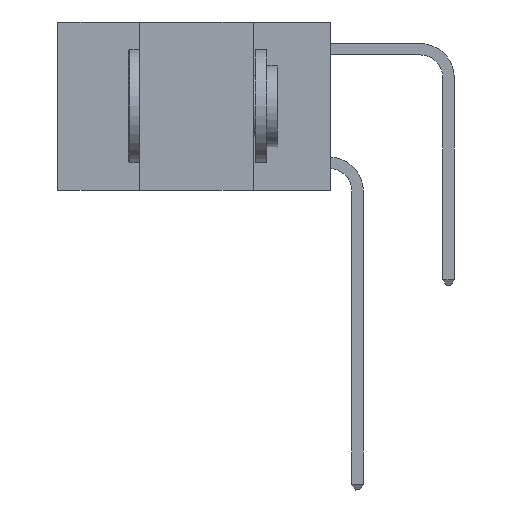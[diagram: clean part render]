
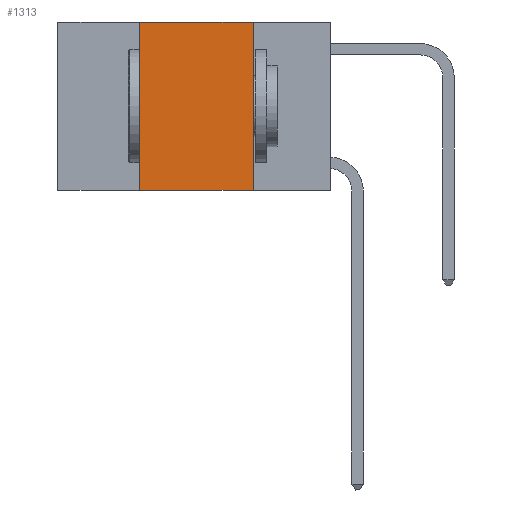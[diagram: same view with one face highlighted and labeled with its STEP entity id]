
A CAD part, left-side view. The second image highlights one B-rep face of the part: STEP entity #1313.
In plain terms, the highlighted planar face has unit normal (-1, 0, 0).
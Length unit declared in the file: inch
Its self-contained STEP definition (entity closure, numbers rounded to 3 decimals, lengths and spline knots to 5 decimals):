
#328 = EDGE_CURVE ( 'NONE', #8473, #8412, #13324, .T. ) ;
#923 = CARTESIAN_POINT ( 'NONE',  ( 0., 0.6, 0. ) ) ;
#1313 = ADVANCED_FACE ( 'NONE', ( #15632 ), #5623, .F. ) ;
#1530 = ORIENTED_EDGE ( 'NONE', *, *, #328, .F. ) ;
#1675 = VECTOR ( 'NONE', #2755, 39.37008 ) ;
#1776 = VECTOR ( 'NONE', #9753, 39.37008 ) ;
#2530 = LINE ( 'NONE', #5169, #1675 ) ;
#2643 = CARTESIAN_POINT ( 'NONE',  ( 0., 0.42, 0. ) ) ;
#2755 = DIRECTION ( 'NONE',  ( 0., 0., 1. ) ) ;
#3214 = DIRECTION ( 'NONE',  ( 0., 0., -1. ) ) ;
#4491 = EDGE_CURVE ( 'NONE', #8412, #13596, #15709, .T. ) ;
#4605 = CARTESIAN_POINT ( 'NONE',  ( 0., 0.17, -0.37 ) ) ;
#5169 = CARTESIAN_POINT ( 'NONE',  ( 0., 0.42, 0. ) ) ;
#5623 = PLANE ( 'NONE',  #15043 ) ;
#6271 = CARTESIAN_POINT ( 'NONE',  ( 0., 0.17, 0. ) ) ;
#6325 = EDGE_CURVE ( 'NONE', #7435, #8473, #2530, .T. ) ;
#6796 = ORIENTED_EDGE ( 'NONE', *, *, #13585, .T. ) ;
#7237 = DIRECTION ( 'NONE',  ( 0., 0., -1. ) ) ;
#7435 = VERTEX_POINT ( 'NONE', #14550 ) ;
#8412 = VERTEX_POINT ( 'NONE', #6271 ) ;
#8473 = VERTEX_POINT ( 'NONE', #2643 ) ;
#9071 = ORIENTED_EDGE ( 'NONE', *, *, #6325, .F. ) ;
#9679 = VECTOR ( 'NONE', #14298, 39.37008 ) ;
#9753 = DIRECTION ( 'NONE',  ( 0., -1., 0. ) ) ;
#11086 = EDGE_LOOP ( 'NONE', ( #11245, #1530, #9071, #6796 ) ) ;
#11245 = ORIENTED_EDGE ( 'NONE', *, *, #4491, .F. ) ;
#12018 = CARTESIAN_POINT ( 'NONE',  ( 0., 0.6, -0.37 ) ) ;
#12074 = CARTESIAN_POINT ( 'NONE',  ( 0., 0.6, 0. ) ) ;
#12173 = LINE ( 'NONE', #12018, #1776 ) ;
#13299 = CARTESIAN_POINT ( 'NONE',  ( 0., 0.17, 0. ) ) ;
#13324 = LINE ( 'NONE', #923, #9679 ) ;
#13585 = EDGE_CURVE ( 'NONE', #7435, #13596, #12173, .T. ) ;
#13596 = VERTEX_POINT ( 'NONE', #4605 ) ;
#14298 = DIRECTION ( 'NONE',  ( 0., -1., 0. ) ) ;
#14550 = CARTESIAN_POINT ( 'NONE',  ( 0., 0.42, -0.37 ) ) ;
#15033 = VECTOR ( 'NONE', #7237, 39.37008 ) ;
#15043 = AXIS2_PLACEMENT_3D ( 'NONE', #12074, #15469, #3214 ) ;
#15469 = DIRECTION ( 'NONE',  ( 1., 0., 0. ) ) ;
#15632 = FACE_OUTER_BOUND ( 'NONE', #11086, .T. ) ;
#15709 = LINE ( 'NONE', #13299, #15033 ) ;
